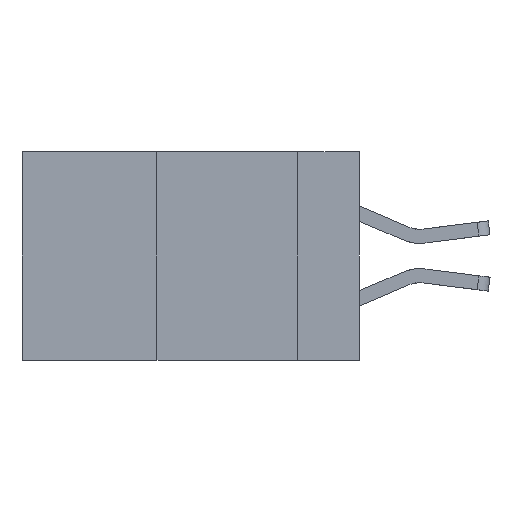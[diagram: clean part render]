
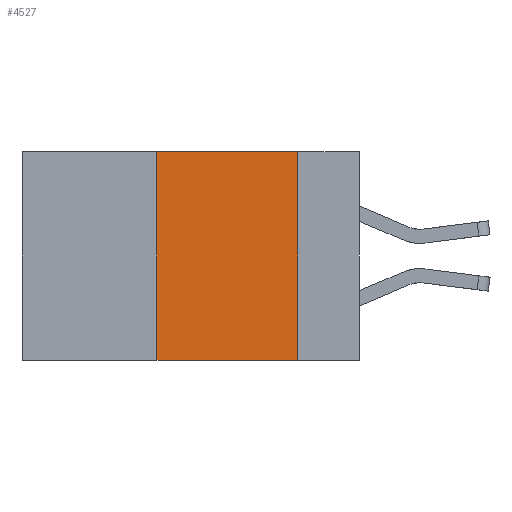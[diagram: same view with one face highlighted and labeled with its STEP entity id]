
A CAD part, left-side view. The second image highlights one B-rep face of the part: STEP entity #4527.
In plain terms, the highlighted planar face has unit normal (-1, 0, 0).
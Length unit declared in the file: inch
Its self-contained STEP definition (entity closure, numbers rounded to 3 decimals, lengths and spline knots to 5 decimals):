
#673 = VERTEX_POINT ( 'NONE', #8346 ) ;
#1302 = VECTOR ( 'NONE', #7805, 39.37008 ) ;
#1583 = EDGE_CURVE ( 'NONE', #8917, #8782, #8831, .T. ) ;
#2055 = DIRECTION ( 'NONE',  ( 0., 0., -1. ) ) ;
#2173 = CARTESIAN_POINT ( 'NONE',  ( 0., 0.36, 0. ) ) ;
#2772 = VECTOR ( 'NONE', #11749, 39.37008 ) ;
#2872 = ORIENTED_EDGE ( 'NONE', *, *, #7374, .T. ) ;
#3113 = CARTESIAN_POINT ( 'NONE',  ( 0., 0.6, 0. ) ) ;
#3884 = LINE ( 'NONE', #5848, #1302 ) ;
#3901 = DIRECTION ( 'NONE',  ( 1., 0., 0. ) ) ;
#3987 = VECTOR ( 'NONE', #6955, 39.37008 ) ;
#4211 = CARTESIAN_POINT ( 'NONE',  ( 0., 0.36, -0.37 ) ) ;
#4337 = CARTESIAN_POINT ( 'NONE',  ( 0., 0.11, 0. ) ) ;
#4527 = ADVANCED_FACE ( 'NONE', ( #5461 ), #7014, .F. ) ;
#5461 = FACE_OUTER_BOUND ( 'NONE', #6803, .T. ) ;
#5848 = CARTESIAN_POINT ( 'NONE',  ( 0., 0.11, 0. ) ) ;
#5941 = EDGE_CURVE ( 'NONE', #11286, #8917, #7978, .T. ) ;
#6036 = ORIENTED_EDGE ( 'NONE', *, *, #11590, .F. ) ;
#6801 = ORIENTED_EDGE ( 'NONE', *, *, #5941, .F. ) ;
#6803 = EDGE_LOOP ( 'NONE', ( #6036, #8899, #6801, #2872 ) ) ;
#6955 = DIRECTION ( 'NONE',  ( 0., 0., 1. ) ) ;
#7014 = PLANE ( 'NONE',  #12240 ) ;
#7374 = EDGE_CURVE ( 'NONE', #11286, #673, #7961, .T. ) ;
#7805 = DIRECTION ( 'NONE',  ( 0., 0., -1. ) ) ;
#7961 = LINE ( 'NONE', #8877, #2772 ) ;
#7978 = LINE ( 'NONE', #2173, #3987 ) ;
#8119 = DIRECTION ( 'NONE',  ( 0., -1., 0. ) ) ;
#8346 = CARTESIAN_POINT ( 'NONE',  ( 0., 0.11, -0.37 ) ) ;
#8525 = VECTOR ( 'NONE', #8119, 39.37008 ) ;
#8782 = VERTEX_POINT ( 'NONE', #4337 ) ;
#8831 = LINE ( 'NONE', #9050, #8525 ) ;
#8877 = CARTESIAN_POINT ( 'NONE',  ( 0., 0.6, -0.37 ) ) ;
#8899 = ORIENTED_EDGE ( 'NONE', *, *, #1583, .F. ) ;
#8917 = VERTEX_POINT ( 'NONE', #9369 ) ;
#9050 = CARTESIAN_POINT ( 'NONE',  ( 0., 0.6, 0. ) ) ;
#9369 = CARTESIAN_POINT ( 'NONE',  ( 0., 0.36, 0. ) ) ;
#11286 = VERTEX_POINT ( 'NONE', #4211 ) ;
#11590 = EDGE_CURVE ( 'NONE', #8782, #673, #3884, .T. ) ;
#11749 = DIRECTION ( 'NONE',  ( 0., -1., 0. ) ) ;
#12240 = AXIS2_PLACEMENT_3D ( 'NONE', #3113, #3901, #2055 ) ;
